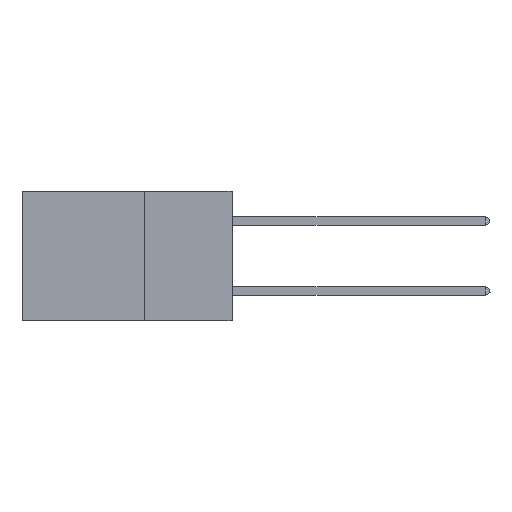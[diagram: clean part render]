
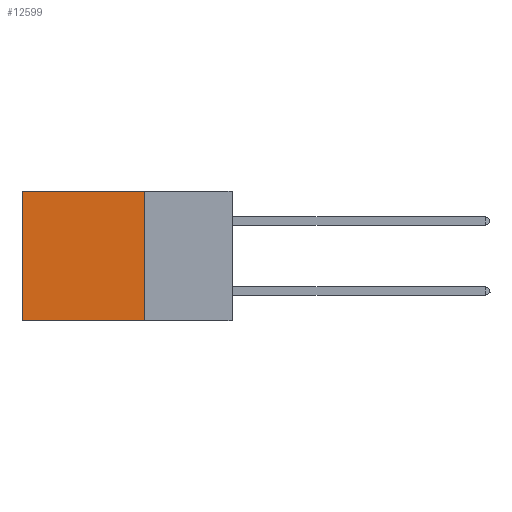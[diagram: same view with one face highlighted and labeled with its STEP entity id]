
A CAD part, left-side view. The second image highlights one B-rep face of the part: STEP entity #12599.
In plain terms, the highlighted planar face has unit normal (-1, 0, 0).
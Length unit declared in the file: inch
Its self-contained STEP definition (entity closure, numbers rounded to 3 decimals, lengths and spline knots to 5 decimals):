
#715 = VERTEX_POINT ( 'NONE', #7744 ) ;
#950 = EDGE_CURVE ( 'NONE', #16152, #715, #7593, .T. ) ;
#2108 = ORIENTED_EDGE ( 'NONE', *, *, #9228, .T. ) ;
#2777 = LINE ( 'NONE', #6197, #16384 ) ;
#3075 = DIRECTION ( 'NONE',  ( 1., 0., 0. ) ) ;
#3637 = CARTESIAN_POINT ( 'NONE',  ( 0.2875, 0.6, 0. ) ) ;
#4244 = CARTESIAN_POINT ( 'NONE',  ( 0.2875, 0.25, -0.37 ) ) ;
#4821 = DIRECTION ( 'NONE',  ( 0., 0., -1. ) ) ;
#4956 = LINE ( 'NONE', #4244, #7493 ) ;
#4990 = VECTOR ( 'NONE', #9916, 39.37008 ) ;
#6113 = AXIS2_PLACEMENT_3D ( 'NONE', #12526, #3075, #12217 ) ;
#6197 = CARTESIAN_POINT ( 'NONE',  ( 0.2875, 0.6, 0. ) ) ;
#6278 = LINE ( 'NONE', #6713, #4990 ) ;
#6539 = CARTESIAN_POINT ( 'NONE',  ( 0.2875, 0.25, 0. ) ) ;
#6713 = CARTESIAN_POINT ( 'NONE',  ( 0.2875, 0.25, 0. ) ) ;
#7493 = VECTOR ( 'NONE', #8236, 39.37008 ) ;
#7593 = LINE ( 'NONE', #12709, #14938 ) ;
#7721 = VERTEX_POINT ( 'NONE', #8750 ) ;
#7744 = CARTESIAN_POINT ( 'NONE',  ( 0.2875, 0.25, -0.37 ) ) ;
#8017 = VERTEX_POINT ( 'NONE', #3637 ) ;
#8236 = DIRECTION ( 'NONE',  ( 0., 1., 0. ) ) ;
#8519 = ORIENTED_EDGE ( 'NONE', *, *, #16029, .T. ) ;
#8750 = CARTESIAN_POINT ( 'NONE',  ( 0.2875, 0.6, -0.37 ) ) ;
#9228 = EDGE_CURVE ( 'NONE', #16152, #8017, #6278, .T. ) ;
#9505 = ORIENTED_EDGE ( 'NONE', *, *, #10213, .F. ) ;
#9916 = DIRECTION ( 'NONE',  ( 0., 1., 0. ) ) ;
#10213 = EDGE_CURVE ( 'NONE', #715, #7721, #4956, .T. ) ;
#10250 = DIRECTION ( 'NONE',  ( 0., 0., -1. ) ) ;
#11266 = PLANE ( 'NONE',  #6113 ) ;
#12217 = DIRECTION ( 'NONE',  ( 0., 0., -1. ) ) ;
#12526 = CARTESIAN_POINT ( 'NONE',  ( 0.2875, 0.25, 0. ) ) ;
#12555 = FACE_OUTER_BOUND ( 'NONE', #15886, .T. ) ;
#12599 = ADVANCED_FACE ( 'NONE', ( #12555 ), #11266, .F. ) ;
#12709 = CARTESIAN_POINT ( 'NONE',  ( 0.2875, 0.25, 0. ) ) ;
#14007 = ORIENTED_EDGE ( 'NONE', *, *, #950, .F. ) ;
#14938 = VECTOR ( 'NONE', #4821, 39.37008 ) ;
#15886 = EDGE_LOOP ( 'NONE', ( #8519, #9505, #14007, #2108 ) ) ;
#16029 = EDGE_CURVE ( 'NONE', #8017, #7721, #2777, .T. ) ;
#16152 = VERTEX_POINT ( 'NONE', #6539 ) ;
#16384 = VECTOR ( 'NONE', #10250, 39.37008 ) ;
